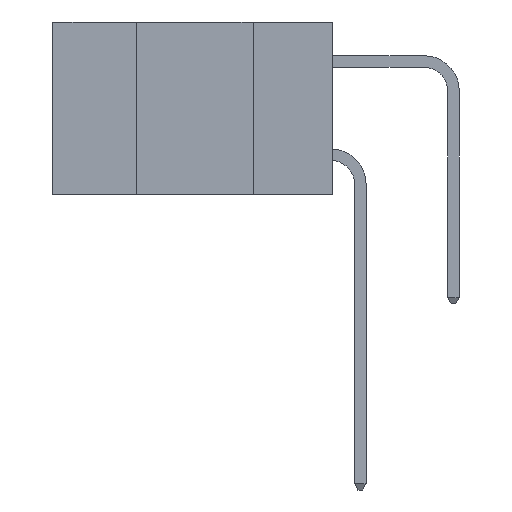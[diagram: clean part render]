
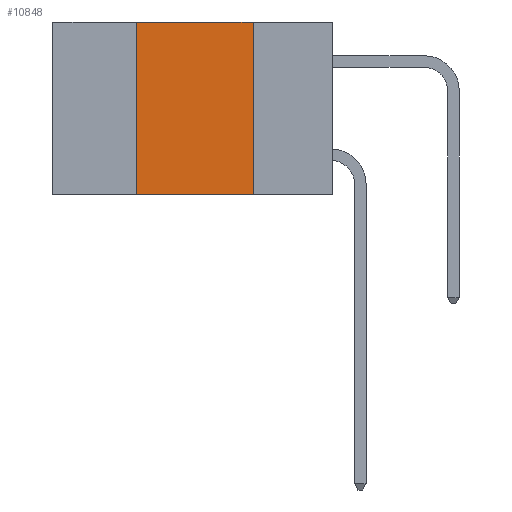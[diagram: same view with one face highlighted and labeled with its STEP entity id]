
A CAD part, left-side view. The second image highlights one B-rep face of the part: STEP entity #10848.
In plain terms, the highlighted planar face has unit normal (-1, 0, 0).
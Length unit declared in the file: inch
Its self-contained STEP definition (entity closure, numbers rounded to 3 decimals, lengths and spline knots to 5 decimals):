
#143 = VECTOR ( 'NONE', #4861, 39.37008 ) ;
#151 = CARTESIAN_POINT ( 'NONE',  ( 0., 0.6, 0. ) ) ;
#210 = EDGE_CURVE ( 'NONE', #10526, #11969, #3692, .T. ) ;
#424 = VECTOR ( 'NONE', #10109, 39.37008 ) ;
#536 = CARTESIAN_POINT ( 'NONE',  ( 0., 0.6, 0. ) ) ;
#537 = CARTESIAN_POINT ( 'NONE',  ( 0., 0.17, -0.37 ) ) ;
#661 = EDGE_CURVE ( 'NONE', #11969, #8309, #6764, .T. ) ;
#675 = DIRECTION ( 'NONE',  ( 0., 0., 1. ) ) ;
#722 = LINE ( 'NONE', #8229, #424 ) ;
#1105 = DIRECTION ( 'NONE',  ( 1., 0., 0. ) ) ;
#1282 = EDGE_CURVE ( 'NONE', #8309, #4806, #10542, .T. ) ;
#1855 = ORIENTED_EDGE ( 'NONE', *, *, #11614, .T. ) ;
#2637 = FACE_OUTER_BOUND ( 'NONE', #9052, .T. ) ;
#3692 = LINE ( 'NONE', #7368, #6845 ) ;
#3742 = CARTESIAN_POINT ( 'NONE',  ( 0., 0.17, -0.37 ) ) ;
#4806 = VERTEX_POINT ( 'NONE', #537 ) ;
#4861 = DIRECTION ( 'NONE',  ( 0., 0., -1. ) ) ;
#5453 = CARTESIAN_POINT ( 'NONE',  ( 0., 0.42, -0.37 ) ) ;
#6764 = LINE ( 'NONE', #536, #11371 ) ;
#6845 = VECTOR ( 'NONE', #675, 39.37008 ) ;
#7368 = CARTESIAN_POINT ( 'NONE',  ( 0., 0.42, -0.37 ) ) ;
#7818 = DIRECTION ( 'NONE',  ( 0., 0., -1. ) ) ;
#7858 = ORIENTED_EDGE ( 'NONE', *, *, #661, .F. ) ;
#8099 = CARTESIAN_POINT ( 'NONE',  ( 0., 0.17, 0. ) ) ;
#8117 = DIRECTION ( 'NONE',  ( 0., -1., 0. ) ) ;
#8144 = ORIENTED_EDGE ( 'NONE', *, *, #210, .F. ) ;
#8229 = CARTESIAN_POINT ( 'NONE',  ( 0., 0.6, -0.37 ) ) ;
#8309 = VERTEX_POINT ( 'NONE', #8099 ) ;
#9052 = EDGE_LOOP ( 'NONE', ( #10032, #7858, #8144, #1855 ) ) ;
#10032 = ORIENTED_EDGE ( 'NONE', *, *, #1282, .F. ) ;
#10109 = DIRECTION ( 'NONE',  ( 0., -1., 0. ) ) ;
#10526 = VERTEX_POINT ( 'NONE', #5453 ) ;
#10542 = LINE ( 'NONE', #3742, #143 ) ;
#10565 = PLANE ( 'NONE',  #11224 ) ;
#10848 = ADVANCED_FACE ( 'NONE', ( #2637 ), #10565, .F. ) ;
#11224 = AXIS2_PLACEMENT_3D ( 'NONE', #151, #1105, #7818 ) ;
#11371 = VECTOR ( 'NONE', #8117, 39.37008 ) ;
#11614 = EDGE_CURVE ( 'NONE', #10526, #4806, #722, .T. ) ;
#11616 = CARTESIAN_POINT ( 'NONE',  ( 0., 0.42, 0. ) ) ;
#11969 = VERTEX_POINT ( 'NONE', #11616 ) ;
